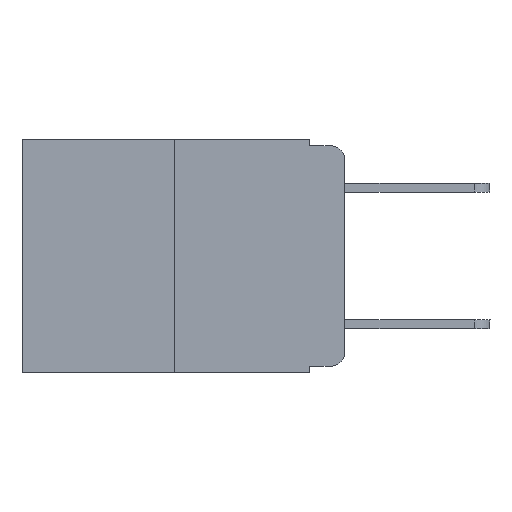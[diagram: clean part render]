
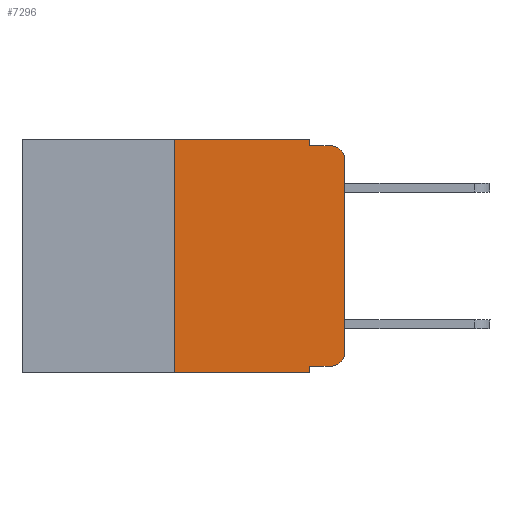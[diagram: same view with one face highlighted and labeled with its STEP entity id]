
A CAD part, left-side view. The second image highlights one B-rep face of the part: STEP entity #7296.
In plain terms, the highlighted planar face has unit normal (-1, 0, 0).
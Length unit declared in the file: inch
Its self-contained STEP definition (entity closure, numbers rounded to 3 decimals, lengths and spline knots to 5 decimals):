
#278 = DIRECTION ( 'NONE',  ( 0., 0., 1. ) ) ;
#319 = CARTESIAN_POINT ( 'NONE',  ( 0., 0.051, -0.01 ) ) ;
#580 = EDGE_CURVE ( 'NONE', #13194, #5579, #1442, .T. ) ;
#757 = VECTOR ( 'NONE', #14756, 39.37008 ) ;
#804 = VECTOR ( 'NONE', #16072, 39.37008 ) ;
#856 = ORIENTED_EDGE ( 'NONE', *, *, #2385, .T. ) ;
#932 = DIRECTION ( 'NONE',  ( 1., 0., 0. ) ) ;
#1042 = ORIENTED_EDGE ( 'NONE', *, *, #4622, .F. ) ;
#1233 = CARTESIAN_POINT ( 'NONE',  ( 0., 0.25, 0. ) ) ;
#1248 = CIRCLE ( 'NONE', #14934, 0.02 ) ;
#1277 = VECTOR ( 'NONE', #13149, 39.37008 ) ;
#1442 = LINE ( 'NONE', #2750, #13029 ) ;
#1681 = CARTESIAN_POINT ( 'NONE',  ( 0., 0.051, -0.01 ) ) ;
#1700 = ORIENTED_EDGE ( 'NONE', *, *, #15696, .F. ) ;
#1835 = DIRECTION ( 'NONE',  ( 0., 0., -1. ) ) ;
#1908 = AXIS2_PLACEMENT_3D ( 'NONE', #9817, #932, #13529 ) ;
#2369 = CARTESIAN_POINT ( 'NONE',  ( 0., 0., -0.313 ) ) ;
#2385 = EDGE_CURVE ( 'NONE', #5579, #7087, #15941, .T. ) ;
#2428 = LINE ( 'NONE', #5296, #5498 ) ;
#2469 = LINE ( 'NONE', #1233, #6169 ) ;
#2647 = VERTEX_POINT ( 'NONE', #4847 ) ;
#2750 = CARTESIAN_POINT ( 'NONE',  ( 0., 0.051, -0.333 ) ) ;
#2906 = EDGE_CURVE ( 'NONE', #9274, #15662, #2469, .T. ) ;
#2910 = CARTESIAN_POINT ( 'NONE',  ( 0., 0., 0. ) ) ;
#3204 = LINE ( 'NONE', #2910, #14290 ) ;
#3251 = EDGE_CURVE ( 'NONE', #7087, #15930, #3204, .T. ) ;
#3389 = FACE_OUTER_BOUND ( 'NONE', #15971, .T. ) ;
#3418 = ORIENTED_EDGE ( 'NONE', *, *, #13552, .F. ) ;
#3581 = VERTEX_POINT ( 'NONE', #319 ) ;
#3713 = LINE ( 'NONE', #5996, #757 ) ;
#3734 = CARTESIAN_POINT ( 'NONE',  ( 0., 0.051, -0.333 ) ) ;
#4422 = EDGE_CURVE ( 'NONE', #15662, #11669, #2428, .T. ) ;
#4487 = LINE ( 'NONE', #13307, #1277 ) ;
#4622 = EDGE_CURVE ( 'NONE', #3581, #8616, #5524, .T. ) ;
#4847 = CARTESIAN_POINT ( 'NONE',  ( 0., 0.051, -0.343 ) ) ;
#4976 = CARTESIAN_POINT ( 'NONE',  ( 0., 0.02, -0.333 ) ) ;
#5198 = EDGE_CURVE ( 'NONE', #9274, #2647, #8560, .T. ) ;
#5296 = CARTESIAN_POINT ( 'NONE',  ( 0., 0.473, 0. ) ) ;
#5498 = VECTOR ( 'NONE', #11242, 39.37008 ) ;
#5524 = LINE ( 'NONE', #1681, #14735 ) ;
#5579 = VERTEX_POINT ( 'NONE', #4976 ) ;
#5996 = CARTESIAN_POINT ( 'NONE',  ( 0., 0.051, 0. ) ) ;
#6169 = VECTOR ( 'NONE', #10041, 39.37008 ) ;
#6429 = DIRECTION ( 'NONE',  ( -1., 0., 0. ) ) ;
#6899 = ORIENTED_EDGE ( 'NONE', *, *, #3251, .T. ) ;
#7087 = VERTEX_POINT ( 'NONE', #2369 ) ;
#7296 = ADVANCED_FACE ( 'NONE', ( #3389 ), #13712, .F. ) ;
#7746 = DIRECTION ( 'NONE',  ( 0., 0., -1. ) ) ;
#7857 = CARTESIAN_POINT ( 'NONE',  ( 0., 0., -0.03 ) ) ;
#8422 = DIRECTION ( 'NONE',  ( -1., 0., 0. ) ) ;
#8560 = LINE ( 'NONE', #14836, #804 ) ;
#8616 = VERTEX_POINT ( 'NONE', #14724 ) ;
#8668 = ORIENTED_EDGE ( 'NONE', *, *, #5198, .T. ) ;
#8825 = AXIS2_PLACEMENT_3D ( 'NONE', #12547, #6429, #7746 ) ;
#9274 = VERTEX_POINT ( 'NONE', #15660 ) ;
#9661 = ORIENTED_EDGE ( 'NONE', *, *, #4422, .F. ) ;
#9817 = CARTESIAN_POINT ( 'NONE',  ( 0., 0.473, 0. ) ) ;
#10041 = DIRECTION ( 'NONE',  ( 0., 0., 1. ) ) ;
#10670 = CARTESIAN_POINT ( 'NONE',  ( 0., 0.25, 0. ) ) ;
#10688 = EDGE_CURVE ( 'NONE', #15930, #8616, #1248, .T. ) ;
#11242 = DIRECTION ( 'NONE',  ( 0., -1., 0. ) ) ;
#11669 = VERTEX_POINT ( 'NONE', #13041 ) ;
#11902 = DIRECTION ( 'NONE',  ( 0., -1., 0. ) ) ;
#12547 = CARTESIAN_POINT ( 'NONE',  ( 0., 0.02, -0.313 ) ) ;
#13029 = VECTOR ( 'NONE', #14123, 39.37008 ) ;
#13041 = CARTESIAN_POINT ( 'NONE',  ( 0., 0.051, 0. ) ) ;
#13080 = ORIENTED_EDGE ( 'NONE', *, *, #10688, .T. ) ;
#13149 = DIRECTION ( 'NONE',  ( 0., 0., -1. ) ) ;
#13194 = VERTEX_POINT ( 'NONE', #3734 ) ;
#13307 = CARTESIAN_POINT ( 'NONE',  ( 0., 0.051, 0. ) ) ;
#13442 = CARTESIAN_POINT ( 'NONE',  ( 0., 0.02, -0.03 ) ) ;
#13529 = DIRECTION ( 'NONE',  ( 0., 0., -1. ) ) ;
#13552 = EDGE_CURVE ( 'NONE', #11669, #3581, #3713, .T. ) ;
#13712 = PLANE ( 'NONE',  #1908 ) ;
#14123 = DIRECTION ( 'NONE',  ( 0., -1., 0. ) ) ;
#14290 = VECTOR ( 'NONE', #278, 39.37008 ) ;
#14414 = ORIENTED_EDGE ( 'NONE', *, *, #2906, .F. ) ;
#14724 = CARTESIAN_POINT ( 'NONE',  ( 0., 0.02, -0.01 ) ) ;
#14735 = VECTOR ( 'NONE', #11902, 39.37008 ) ;
#14756 = DIRECTION ( 'NONE',  ( 0., 0., -1. ) ) ;
#14836 = CARTESIAN_POINT ( 'NONE',  ( 0., 0.473, -0.343 ) ) ;
#14934 = AXIS2_PLACEMENT_3D ( 'NONE', #13442, #8422, #1835 ) ;
#15660 = CARTESIAN_POINT ( 'NONE',  ( 0., 0.25, -0.343 ) ) ;
#15662 = VERTEX_POINT ( 'NONE', #10670 ) ;
#15696 = EDGE_CURVE ( 'NONE', #13194, #2647, #4487, .T. ) ;
#15786 = ORIENTED_EDGE ( 'NONE', *, *, #580, .T. ) ;
#15930 = VERTEX_POINT ( 'NONE', #7857 ) ;
#15941 = CIRCLE ( 'NONE', #8825, 0.02 ) ;
#15971 = EDGE_LOOP ( 'NONE', ( #6899, #13080, #1042, #3418, #9661, #14414, #8668, #1700, #15786, #856 ) ) ;
#16072 = DIRECTION ( 'NONE',  ( 0., -1., 0. ) ) ;
